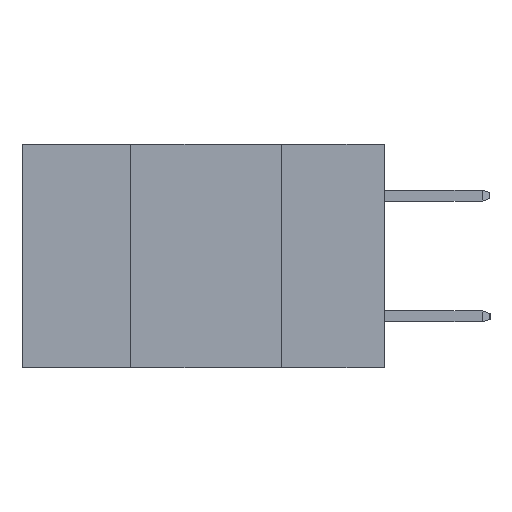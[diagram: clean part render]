
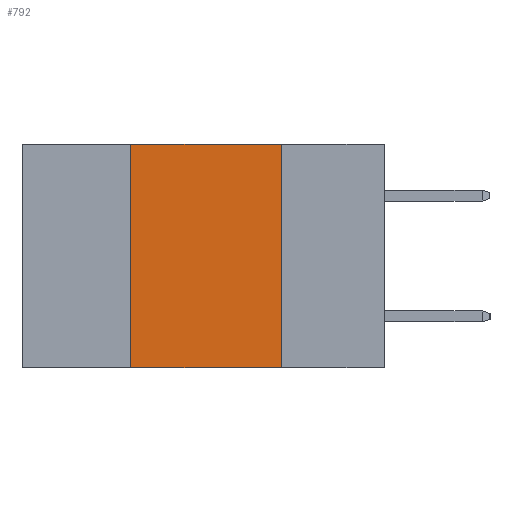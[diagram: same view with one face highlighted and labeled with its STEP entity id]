
A CAD part, left-side view. The second image highlights one B-rep face of the part: STEP entity #792.
In plain terms, the highlighted planar face has unit normal (-1, 0, 0).
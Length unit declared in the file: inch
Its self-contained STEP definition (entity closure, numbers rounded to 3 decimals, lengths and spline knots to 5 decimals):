
#3 = LINE ( 'NONE', #15062, #6506 ) ;
#689 = VECTOR ( 'NONE', #5721, 39.37008 ) ;
#711 = AXIS2_PLACEMENT_3D ( 'NONE', #10870, #9710, #9594 ) ;
#792 = ADVANCED_FACE ( 'NONE', ( #14253 ), #9881, .F. ) ;
#2086 = ORIENTED_EDGE ( 'NONE', *, *, #13069, .F. ) ;
#2166 = CARTESIAN_POINT ( 'NONE',  ( 0., 0.42, -0.37 ) ) ;
#2334 = CARTESIAN_POINT ( 'NONE',  ( 0., 0.17, 0. ) ) ;
#2415 = CARTESIAN_POINT ( 'NONE',  ( 0., 0.17, -0.37 ) ) ;
#2465 = DIRECTION ( 'NONE',  ( 0., 0., -1. ) ) ;
#3906 = VECTOR ( 'NONE', #2465, 39.37008 ) ;
#4598 = LINE ( 'NONE', #8314, #11544 ) ;
#4765 = EDGE_CURVE ( 'NONE', #12083, #7714, #3, .T. ) ;
#5209 = ORIENTED_EDGE ( 'NONE', *, *, #4765, .F. ) ;
#5692 = CARTESIAN_POINT ( 'NONE',  ( 0., 0.42, 0. ) ) ;
#5721 = DIRECTION ( 'NONE',  ( 0., 0., 1. ) ) ;
#5994 = CARTESIAN_POINT ( 'NONE',  ( 0., 0.42, -0.37 ) ) ;
#6095 = CARTESIAN_POINT ( 'NONE',  ( 0., 0.17, -0.37 ) ) ;
#6506 = VECTOR ( 'NONE', #15238, 39.37008 ) ;
#6962 = EDGE_CURVE ( 'NONE', #14456, #13090, #4598, .T. ) ;
#7714 = VERTEX_POINT ( 'NONE', #2334 ) ;
#8314 = CARTESIAN_POINT ( 'NONE',  ( 0., 0.6, -0.37 ) ) ;
#8666 = DIRECTION ( 'NONE',  ( 0., -1., 0. ) ) ;
#8816 = EDGE_LOOP ( 'NONE', ( #13795, #5209, #2086, #9068 ) ) ;
#9068 = ORIENTED_EDGE ( 'NONE', *, *, #6962, .T. ) ;
#9594 = DIRECTION ( 'NONE',  ( 0., 0., -1. ) ) ;
#9710 = DIRECTION ( 'NONE',  ( 1., 0., 0. ) ) ;
#9881 = PLANE ( 'NONE',  #711 ) ;
#10472 = LINE ( 'NONE', #2415, #3906 ) ;
#10670 = LINE ( 'NONE', #5994, #689 ) ;
#10870 = CARTESIAN_POINT ( 'NONE',  ( 0., 0.6, 0. ) ) ;
#11544 = VECTOR ( 'NONE', #8666, 39.37008 ) ;
#12083 = VERTEX_POINT ( 'NONE', #5692 ) ;
#12839 = EDGE_CURVE ( 'NONE', #7714, #13090, #10472, .T. ) ;
#13069 = EDGE_CURVE ( 'NONE', #14456, #12083, #10670, .T. ) ;
#13090 = VERTEX_POINT ( 'NONE', #6095 ) ;
#13795 = ORIENTED_EDGE ( 'NONE', *, *, #12839, .F. ) ;
#14253 = FACE_OUTER_BOUND ( 'NONE', #8816, .T. ) ;
#14456 = VERTEX_POINT ( 'NONE', #2166 ) ;
#15062 = CARTESIAN_POINT ( 'NONE',  ( 0., 0.6, 0. ) ) ;
#15238 = DIRECTION ( 'NONE',  ( 0., -1., 0. ) ) ;
